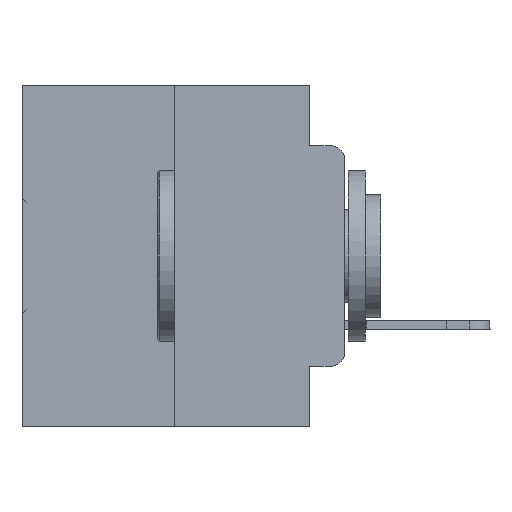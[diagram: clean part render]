
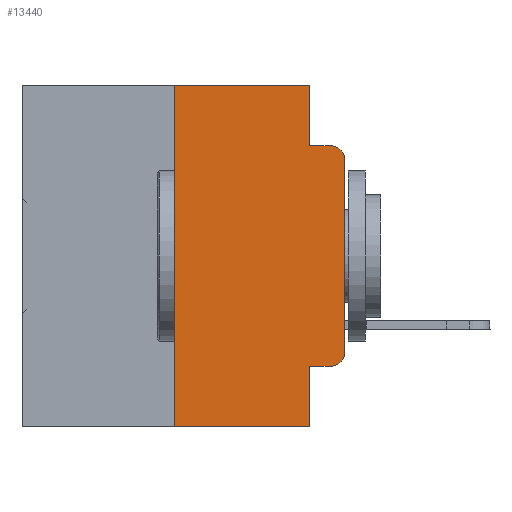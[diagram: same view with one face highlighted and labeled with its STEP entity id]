
A CAD part, left-side view. The second image highlights one B-rep face of the part: STEP entity #13440.
In plain terms, the highlighted planar face has unit normal (-1, 0, 0).
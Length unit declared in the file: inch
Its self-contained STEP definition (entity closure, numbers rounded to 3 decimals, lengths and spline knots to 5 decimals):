
#13 = EDGE_CURVE ( 'NONE', #4453, #32695, #31429, .T. ) ;
#597 = CARTESIAN_POINT ( 'NONE',  ( 0., 0.051, 0. ) ) ;
#724 = VECTOR ( 'NONE', #11737, 39.37008 ) ;
#1143 = CARTESIAN_POINT ( 'NONE',  ( 0., 0.02, -0.1085 ) ) ;
#2338 = EDGE_CURVE ( 'NONE', #8103, #31305, #21393, .T. ) ;
#3192 = CARTESIAN_POINT ( 'NONE',  ( 0., 0.02, -0.3915 ) ) ;
#3478 = DIRECTION ( 'NONE',  ( 0., -1., 0. ) ) ;
#4453 = VERTEX_POINT ( 'NONE', #19197 ) ;
#4974 = CARTESIAN_POINT ( 'NONE',  ( 0., 0.051, -0.0885 ) ) ;
#5178 = CARTESIAN_POINT ( 'NONE',  ( 0., 0.25, -0.5 ) ) ;
#5205 = ORIENTED_EDGE ( 'NONE', *, *, #8962, .F. ) ;
#5967 = DIRECTION ( 'NONE',  ( -1., 0., 0. ) ) ;
#6436 = LINE ( 'NONE', #17050, #29501 ) ;
#6523 = VERTEX_POINT ( 'NONE', #4974 ) ;
#6539 = DIRECTION ( 'NONE',  ( 0., -1., 0. ) ) ;
#6735 = VERTEX_POINT ( 'NONE', #7267 ) ;
#6826 = VECTOR ( 'NONE', #13944, 39.37008 ) ;
#7267 = CARTESIAN_POINT ( 'NONE',  ( 0., 0., -0.3915 ) ) ;
#8103 = VERTEX_POINT ( 'NONE', #20014 ) ;
#8393 = CARTESIAN_POINT ( 'NONE',  ( 0., 0.25, 0. ) ) ;
#8962 = EDGE_CURVE ( 'NONE', #19550, #31031, #20154, .T. ) ;
#9013 = EDGE_CURVE ( 'NONE', #30945, #32695, #6436, .T. ) ;
#9533 = CARTESIAN_POINT ( 'NONE',  ( 0., 0.02, -0.0885 ) ) ;
#9534 = CARTESIAN_POINT ( 'NONE',  ( 0., 0.473, 0. ) ) ;
#9760 = PLANE ( 'NONE',  #17647 ) ;
#10874 = LINE ( 'NONE', #8393, #22179 ) ;
#11075 = CIRCLE ( 'NONE', #21774, 0.02 ) ;
#11121 = AXIS2_PLACEMENT_3D ( 'NONE', #1143, #5967, #21801 ) ;
#11482 = CARTESIAN_POINT ( 'NONE',  ( 0., 0.051, 0. ) ) ;
#11737 = DIRECTION ( 'NONE',  ( 0., 0., -1. ) ) ;
#12326 = DIRECTION ( 'NONE',  ( 0., 0., -1. ) ) ;
#13440 = ADVANCED_FACE ( 'NONE', ( #19077 ), #9760, .F. ) ;
#13686 = DIRECTION ( 'NONE',  ( 0., 0., 1. ) ) ;
#13944 = DIRECTION ( 'NONE',  ( 0., 0., -1. ) ) ;
#14504 = LINE ( 'NONE', #11482, #6826 ) ;
#16970 = LINE ( 'NONE', #32395, #18135 ) ;
#17050 = CARTESIAN_POINT ( 'NONE',  ( 0., 0.473, -0.5 ) ) ;
#17647 = AXIS2_PLACEMENT_3D ( 'NONE', #9534, #19742, #12326 ) ;
#17999 = EDGE_CURVE ( 'NONE', #31031, #6523, #14504, .T. ) ;
#18135 = VECTOR ( 'NONE', #6539, 39.37008 ) ;
#18781 = VECTOR ( 'NONE', #13686, 39.37008 ) ;
#18860 = CARTESIAN_POINT ( 'NONE',  ( 0., 0., 0. ) ) ;
#18935 = EDGE_LOOP ( 'NONE', ( #21036, #27621, #24113, #19071, #5205, #28542, #19433, #21178, #19515, #28154 ) ) ;
#19071 = ORIENTED_EDGE ( 'NONE', *, *, #17999, .F. ) ;
#19077 = FACE_OUTER_BOUND ( 'NONE', #18935, .T. ) ;
#19099 = DIRECTION ( 'NONE',  ( -1., 0., 0. ) ) ;
#19126 = VERTEX_POINT ( 'NONE', #20872 ) ;
#19197 = CARTESIAN_POINT ( 'NONE',  ( 0., 0.051, -0.4115 ) ) ;
#19433 = ORIENTED_EDGE ( 'NONE', *, *, #9013, .T. ) ;
#19515 = ORIENTED_EDGE ( 'NONE', *, *, #25691, .T. ) ;
#19550 = VERTEX_POINT ( 'NONE', #33042 ) ;
#19742 = DIRECTION ( 'NONE',  ( 1., 0., 0. ) ) ;
#20014 = CARTESIAN_POINT ( 'NONE',  ( 0., 0., -0.1085 ) ) ;
#20154 = LINE ( 'NONE', #22255, #23458 ) ;
#20872 = CARTESIAN_POINT ( 'NONE',  ( 0., 0.02, -0.4115 ) ) ;
#21036 = ORIENTED_EDGE ( 'NONE', *, *, #21528, .T. ) ;
#21178 = ORIENTED_EDGE ( 'NONE', *, *, #13, .F. ) ;
#21393 = CIRCLE ( 'NONE', #11121, 0.02 ) ;
#21528 = EDGE_CURVE ( 'NONE', #6735, #8103, #25675, .T. ) ;
#21774 = AXIS2_PLACEMENT_3D ( 'NONE', #3192, #19099, #23900 ) ;
#21801 = DIRECTION ( 'NONE',  ( 0., 0., -1. ) ) ;
#22179 = VECTOR ( 'NONE', #31737, 39.37008 ) ;
#22255 = CARTESIAN_POINT ( 'NONE',  ( 0., 0.473, 0. ) ) ;
#22492 = CARTESIAN_POINT ( 'NONE',  ( 0., 0.051, -0.4115 ) ) ;
#23458 = VECTOR ( 'NONE', #3478, 39.37008 ) ;
#23529 = EDGE_CURVE ( 'NONE', #19126, #6735, #11075, .T. ) ;
#23900 = DIRECTION ( 'NONE',  ( 0., 0., -1. ) ) ;
#24113 = ORIENTED_EDGE ( 'NONE', *, *, #28218, .F. ) ;
#25189 = DIRECTION ( 'NONE',  ( 0., -1., 0. ) ) ;
#25675 = LINE ( 'NONE', #18860, #18781 ) ;
#25691 = EDGE_CURVE ( 'NONE', #4453, #19126, #27654, .T. ) ;
#27621 = ORIENTED_EDGE ( 'NONE', *, *, #2338, .T. ) ;
#27654 = LINE ( 'NONE', #22492, #30118 ) ;
#28154 = ORIENTED_EDGE ( 'NONE', *, *, #23529, .T. ) ;
#28218 = EDGE_CURVE ( 'NONE', #6523, #31305, #16970, .T. ) ;
#28542 = ORIENTED_EDGE ( 'NONE', *, *, #29390, .F. ) ;
#29129 = DIRECTION ( 'NONE',  ( 0., -1., 0. ) ) ;
#29390 = EDGE_CURVE ( 'NONE', #30945, #19550, #10874, .T. ) ;
#29501 = VECTOR ( 'NONE', #29129, 39.37008 ) ;
#30118 = VECTOR ( 'NONE', #25189, 39.37008 ) ;
#30131 = CARTESIAN_POINT ( 'NONE',  ( 0., 0.051, 0. ) ) ;
#30945 = VERTEX_POINT ( 'NONE', #5178 ) ;
#31031 = VERTEX_POINT ( 'NONE', #597 ) ;
#31305 = VERTEX_POINT ( 'NONE', #9533 ) ;
#31367 = CARTESIAN_POINT ( 'NONE',  ( 0., 0.051, -0.5 ) ) ;
#31429 = LINE ( 'NONE', #30131, #724 ) ;
#31737 = DIRECTION ( 'NONE',  ( 0., 0., 1. ) ) ;
#32395 = CARTESIAN_POINT ( 'NONE',  ( 0., 0.051, -0.0885 ) ) ;
#32695 = VERTEX_POINT ( 'NONE', #31367 ) ;
#33042 = CARTESIAN_POINT ( 'NONE',  ( 0., 0.25, 0. ) ) ;
